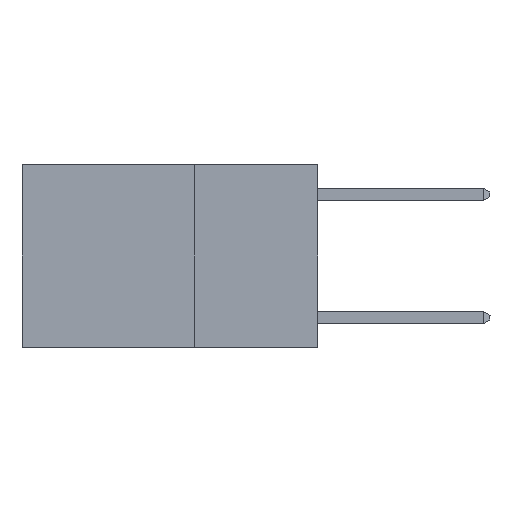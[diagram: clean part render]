
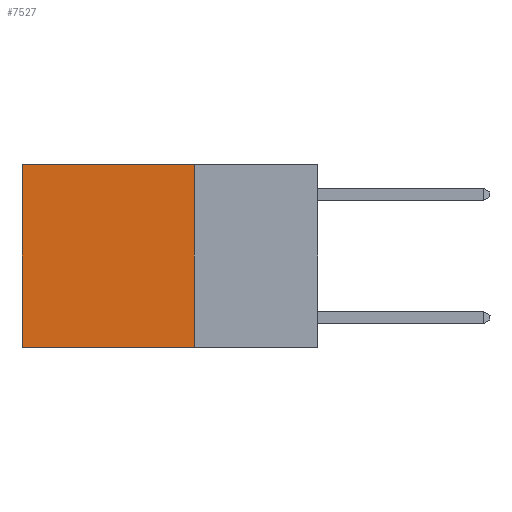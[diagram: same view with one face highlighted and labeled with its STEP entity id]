
A CAD part, left-side view. The second image highlights one B-rep face of the part: STEP entity #7527.
In plain terms, the highlighted planar face has unit normal (-1, 0, 0).
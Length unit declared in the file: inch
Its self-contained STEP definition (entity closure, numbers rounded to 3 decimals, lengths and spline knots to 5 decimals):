
#432 = CARTESIAN_POINT ( 'NONE',  ( 0.2625, 0.25, 0. ) ) ;
#2509 = LINE ( 'NONE', #24198, #14539 ) ;
#2905 = DIRECTION ( 'NONE',  ( 0., 0., -1. ) ) ;
#3422 = EDGE_LOOP ( 'NONE', ( #7763, #8888, #23323, #17392 ) ) ;
#3886 = DIRECTION ( 'NONE',  ( 0., 1., 0. ) ) ;
#6384 = VECTOR ( 'NONE', #30430, 39.37008 ) ;
#7139 = LINE ( 'NONE', #9516, #6384 ) ;
#7527 = ADVANCED_FACE ( 'NONE', ( #21250 ), #10164, .F. ) ;
#7763 = ORIENTED_EDGE ( 'NONE', *, *, #11497, .T. ) ;
#8888 = ORIENTED_EDGE ( 'NONE', *, *, #21322, .F. ) ;
#9516 = CARTESIAN_POINT ( 'NONE',  ( 0.2625, 0.6, 0. ) ) ;
#10164 = PLANE ( 'NONE',  #20138 ) ;
#11313 = CARTESIAN_POINT ( 'NONE',  ( 0.2625, 0.6, 0. ) ) ;
#11497 = EDGE_CURVE ( 'NONE', #14999, #19001, #7139, .T. ) ;
#11664 = EDGE_CURVE ( 'NONE', #24950, #14999, #2509, .T. ) ;
#11769 = VECTOR ( 'NONE', #27005, 39.37008 ) ;
#12480 = DIRECTION ( 'NONE',  ( 0., 1., 0. ) ) ;
#12776 = CARTESIAN_POINT ( 'NONE',  ( 0.2625, 0.25, 0. ) ) ;
#14539 = VECTOR ( 'NONE', #12480, 39.37008 ) ;
#14999 = VERTEX_POINT ( 'NONE', #11313 ) ;
#15832 = CARTESIAN_POINT ( 'NONE',  ( 0.2625, 0.25, -0.37 ) ) ;
#17258 = DIRECTION ( 'NONE',  ( 1., 0., 0. ) ) ;
#17392 = ORIENTED_EDGE ( 'NONE', *, *, #11664, .T. ) ;
#18034 = LINE ( 'NONE', #22377, #11769 ) ;
#19001 = VERTEX_POINT ( 'NONE', #28206 ) ;
#20138 = AXIS2_PLACEMENT_3D ( 'NONE', #432, #17258, #2905 ) ;
#21250 = FACE_OUTER_BOUND ( 'NONE', #3422, .T. ) ;
#21322 = EDGE_CURVE ( 'NONE', #30006, #19001, #30497, .T. ) ;
#21743 = CARTESIAN_POINT ( 'NONE',  ( 0.2625, 0.25, -0.37 ) ) ;
#22377 = CARTESIAN_POINT ( 'NONE',  ( 0.2625, 0.25, 0. ) ) ;
#23323 = ORIENTED_EDGE ( 'NONE', *, *, #26940, .F. ) ;
#23762 = VECTOR ( 'NONE', #3886, 39.37008 ) ;
#24198 = CARTESIAN_POINT ( 'NONE',  ( 0.2625, 0.25, 0. ) ) ;
#24950 = VERTEX_POINT ( 'NONE', #12776 ) ;
#26940 = EDGE_CURVE ( 'NONE', #24950, #30006, #18034, .T. ) ;
#27005 = DIRECTION ( 'NONE',  ( 0., 0., -1. ) ) ;
#28206 = CARTESIAN_POINT ( 'NONE',  ( 0.2625, 0.6, -0.37 ) ) ;
#30006 = VERTEX_POINT ( 'NONE', #21743 ) ;
#30430 = DIRECTION ( 'NONE',  ( 0., 0., -1. ) ) ;
#30497 = LINE ( 'NONE', #15832, #23762 ) ;
